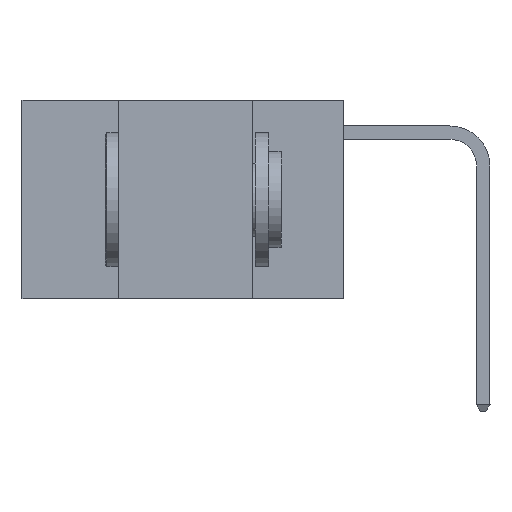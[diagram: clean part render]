
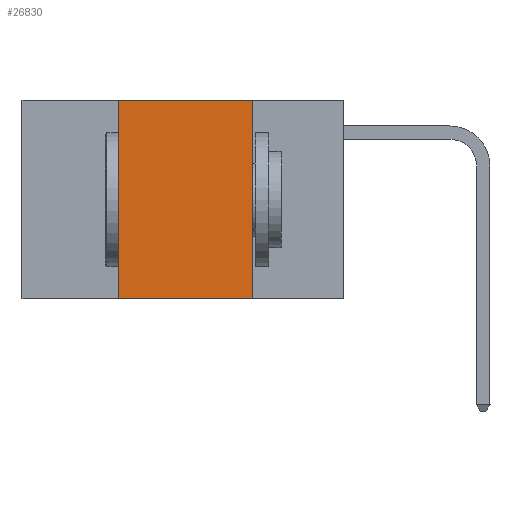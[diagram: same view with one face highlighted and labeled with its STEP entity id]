
A CAD part, left-side view. The second image highlights one B-rep face of the part: STEP entity #26830.
In plain terms, the highlighted planar face has unit normal (-1, 0, 0).
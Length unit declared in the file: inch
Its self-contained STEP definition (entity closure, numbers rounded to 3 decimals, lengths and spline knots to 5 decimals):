
#304 = VERTEX_POINT ( 'NONE', #24330 ) ;
#1952 = EDGE_CURVE ( 'NONE', #9355, #7701, #22054, .T. ) ;
#2361 = VECTOR ( 'NONE', #17426, 39.37008 ) ;
#2887 = VECTOR ( 'NONE', #9075, 39.37008 ) ;
#3651 = ORIENTED_EDGE ( 'NONE', *, *, #1952, .F. ) ;
#5028 = CARTESIAN_POINT ( 'NONE',  ( 0., 0.6, 0. ) ) ;
#6175 = CARTESIAN_POINT ( 'NONE',  ( 0., 0.17, -0.37 ) ) ;
#6920 = ORIENTED_EDGE ( 'NONE', *, *, #23244, .F. ) ;
#7081 = EDGE_LOOP ( 'NONE', ( #3651, #6920, #23963, #25589 ) ) ;
#7514 = PLANE ( 'NONE',  #14667 ) ;
#7701 = VERTEX_POINT ( 'NONE', #6175 ) ;
#8243 = EDGE_CURVE ( 'NONE', #23170, #7701, #10912, .T. ) ;
#8815 = LINE ( 'NONE', #5028, #2361 ) ;
#9075 = DIRECTION ( 'NONE',  ( 0., -1., 0. ) ) ;
#9355 = VERTEX_POINT ( 'NONE', #22277 ) ;
#9460 = VECTOR ( 'NONE', #15415, 39.37008 ) ;
#9483 = CARTESIAN_POINT ( 'NONE',  ( 0., 0.6, 0. ) ) ;
#10912 = LINE ( 'NONE', #19646, #2887 ) ;
#13450 = DIRECTION ( 'NONE',  ( 1., 0., 0. ) ) ;
#13525 = EDGE_CURVE ( 'NONE', #23170, #304, #14696, .T. ) ;
#14667 = AXIS2_PLACEMENT_3D ( 'NONE', #9483, #13450, #17943 ) ;
#14696 = LINE ( 'NONE', #25822, #25549 ) ;
#15415 = DIRECTION ( 'NONE',  ( 0., 0., -1. ) ) ;
#15835 = FACE_OUTER_BOUND ( 'NONE', #7081, .T. ) ;
#17426 = DIRECTION ( 'NONE',  ( 0., -1., 0. ) ) ;
#17943 = DIRECTION ( 'NONE',  ( 0., 0., -1. ) ) ;
#19646 = CARTESIAN_POINT ( 'NONE',  ( 0., 0.6, -0.37 ) ) ;
#22054 = LINE ( 'NONE', #25860, #9460 ) ;
#22277 = CARTESIAN_POINT ( 'NONE',  ( 0., 0.17, 0. ) ) ;
#23170 = VERTEX_POINT ( 'NONE', #26599 ) ;
#23244 = EDGE_CURVE ( 'NONE', #304, #9355, #8815, .T. ) ;
#23963 = ORIENTED_EDGE ( 'NONE', *, *, #13525, .F. ) ;
#24330 = CARTESIAN_POINT ( 'NONE',  ( 0., 0.42, 0. ) ) ;
#25541 = DIRECTION ( 'NONE',  ( 0., 0., 1. ) ) ;
#25549 = VECTOR ( 'NONE', #25541, 39.37008 ) ;
#25589 = ORIENTED_EDGE ( 'NONE', *, *, #8243, .T. ) ;
#25822 = CARTESIAN_POINT ( 'NONE',  ( 0., 0.42, 0. ) ) ;
#25860 = CARTESIAN_POINT ( 'NONE',  ( 0., 0.17, 0. ) ) ;
#26599 = CARTESIAN_POINT ( 'NONE',  ( 0., 0.42, -0.37 ) ) ;
#26830 = ADVANCED_FACE ( 'NONE', ( #15835 ), #7514, .F. ) ;
